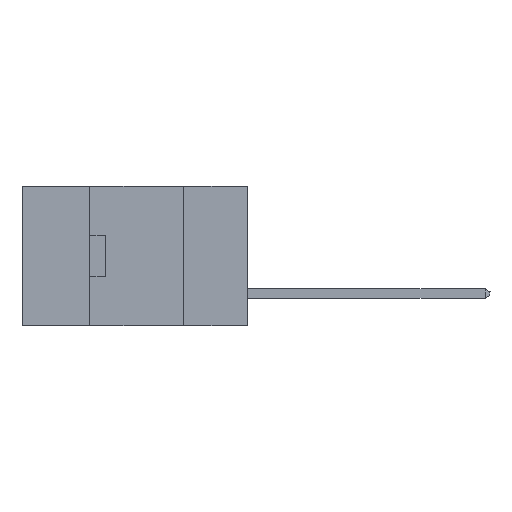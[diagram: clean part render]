
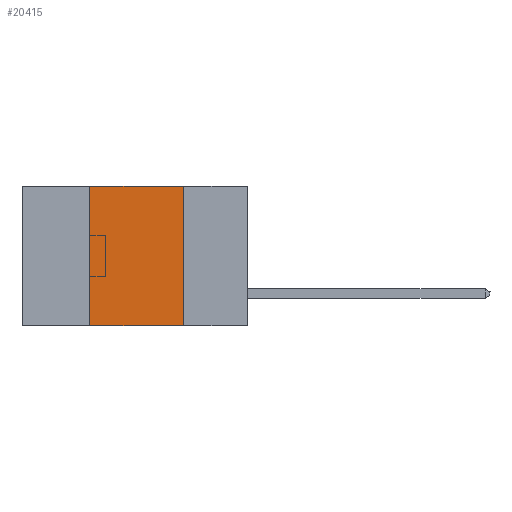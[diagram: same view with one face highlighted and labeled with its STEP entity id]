
A CAD part, left-side view. The second image highlights one B-rep face of the part: STEP entity #20415.
In plain terms, the highlighted planar face has unit normal (-1, 0, 0).
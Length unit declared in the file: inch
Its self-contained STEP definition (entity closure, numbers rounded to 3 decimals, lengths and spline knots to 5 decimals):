
#1783 = VECTOR ( 'NONE', #7884, 39.37008 ) ;
#1954 = VERTEX_POINT ( 'NONE', #13622 ) ;
#2260 = CARTESIAN_POINT ( 'NONE',  ( 0., 0.6, -0.37 ) ) ;
#2936 = DIRECTION ( 'NONE',  ( 0., -1., 0. ) ) ;
#3048 = VERTEX_POINT ( 'NONE', #8080 ) ;
#5069 = EDGE_CURVE ( 'NONE', #3048, #10649, #8159, .T. ) ;
#5128 = ORIENTED_EDGE ( 'NONE', *, *, #23555, .T. ) ;
#5270 = LINE ( 'NONE', #25773, #17748 ) ;
#6390 = LINE ( 'NONE', #8879, #7104 ) ;
#7104 = VECTOR ( 'NONE', #19018, 39.37008 ) ;
#7884 = DIRECTION ( 'NONE',  ( 0., 0., 1. ) ) ;
#8080 = CARTESIAN_POINT ( 'NONE',  ( 0., 0.42, -0.37 ) ) ;
#8159 = LINE ( 'NONE', #16075, #1783 ) ;
#8879 = CARTESIAN_POINT ( 'NONE',  ( 0., 0.17, -0.37 ) ) ;
#9603 = DIRECTION ( 'NONE',  ( 0., 0., -1. ) ) ;
#10019 = ORIENTED_EDGE ( 'NONE', *, *, #26042, .F. ) ;
#10639 = DIRECTION ( 'NONE',  ( 0., -1., 0. ) ) ;
#10649 = VERTEX_POINT ( 'NONE', #26995 ) ;
#11834 = VECTOR ( 'NONE', #10639, 39.37008 ) ;
#13066 = CARTESIAN_POINT ( 'NONE',  ( 0., 0.17, 0. ) ) ;
#13622 = CARTESIAN_POINT ( 'NONE',  ( 0., 0.17, -0.37 ) ) ;
#14487 = ORIENTED_EDGE ( 'NONE', *, *, #17935, .F. ) ;
#16008 = FACE_OUTER_BOUND ( 'NONE', #26632, .T. ) ;
#16075 = CARTESIAN_POINT ( 'NONE',  ( 0., 0.42, -0.37 ) ) ;
#17748 = VECTOR ( 'NONE', #2936, 39.37008 ) ;
#17769 = PLANE ( 'NONE',  #19923 ) ;
#17935 = EDGE_CURVE ( 'NONE', #10649, #18004, #5270, .T. ) ;
#18004 = VERTEX_POINT ( 'NONE', #13066 ) ;
#18021 = DIRECTION ( 'NONE',  ( 1., 0., 0. ) ) ;
#19018 = DIRECTION ( 'NONE',  ( 0., 0., -1. ) ) ;
#19923 = AXIS2_PLACEMENT_3D ( 'NONE', #26122, #18021, #9603 ) ;
#20415 = ADVANCED_FACE ( 'NONE', ( #16008 ), #17769, .F. ) ;
#22605 = LINE ( 'NONE', #2260, #11834 ) ;
#23555 = EDGE_CURVE ( 'NONE', #3048, #1954, #22605, .T. ) ;
#24414 = ORIENTED_EDGE ( 'NONE', *, *, #5069, .F. ) ;
#25773 = CARTESIAN_POINT ( 'NONE',  ( 0., 0.6, 0. ) ) ;
#26042 = EDGE_CURVE ( 'NONE', #18004, #1954, #6390, .T. ) ;
#26122 = CARTESIAN_POINT ( 'NONE',  ( 0., 0.6, 0. ) ) ;
#26632 = EDGE_LOOP ( 'NONE', ( #10019, #14487, #24414, #5128 ) ) ;
#26995 = CARTESIAN_POINT ( 'NONE',  ( 0., 0.42, 0. ) ) ;
